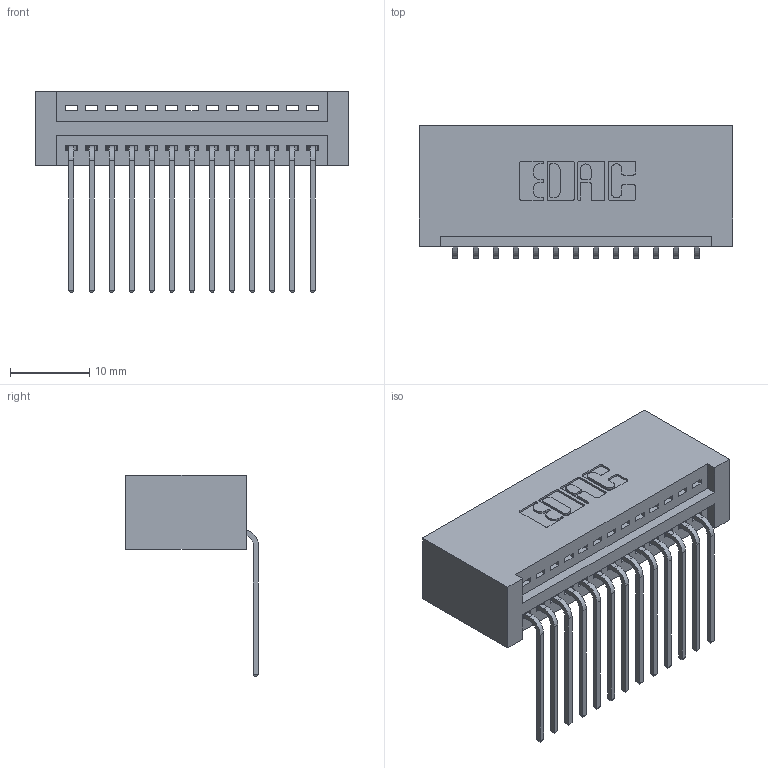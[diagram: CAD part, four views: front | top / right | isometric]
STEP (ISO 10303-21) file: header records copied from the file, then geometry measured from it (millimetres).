
FILE_DESCRIPTION (( 'STEP AP203' ), '1' );
FILE_NAME ('395-013-559-101.STEP', '2018-11-05T21:52:49', ( '' ), ( '' ), 'SwSTEP 2.0', 'SolidWorks 2016', '' );
FILE_SCHEMA (( 'CONFIG_CONTROL_DESIGN' ));
Length unit declared in the file: inch
Products named in the file (3): 345 Part_No Mounting Lugs; 395-013-559-101; 345-292-001_558 559 Tail - 1
Assembly tree (14 placements, depth 2):
  395-013-559-101
    345 Part_No Mounting Lugs
    345-292-001_558 559 Tail - 1  x13
Bounding box: 39.62 x 16.75 x 25.53 mm (x, y, z)
Volume: 4153.6 mm3; surface area: 5570.3 mm2
Topology: 14 solids, 14 shells, 898 faces, 2683 edges, 1770 vertices
Faces by surface type: plane 622, cylinder 276
Entity records: 13495 total; most frequent: CARTESIAN_POINT 2347, ORIENTED_EDGE 2294, DIRECTION 2085, EDGE_CURVE 1147, LINE 971, VECTOR 971, VERTEX_POINT 762, AXIS2_PLACEMENT_3D 557
